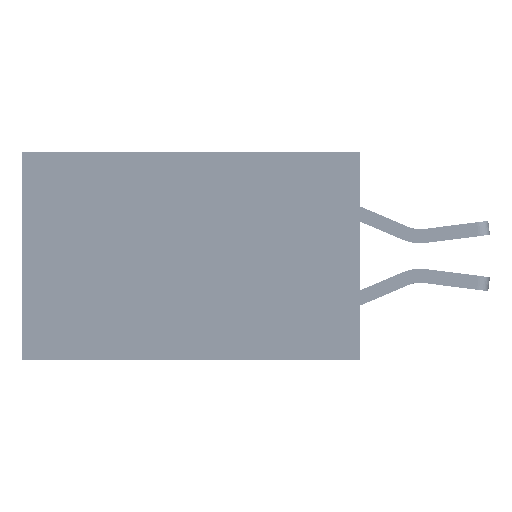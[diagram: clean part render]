
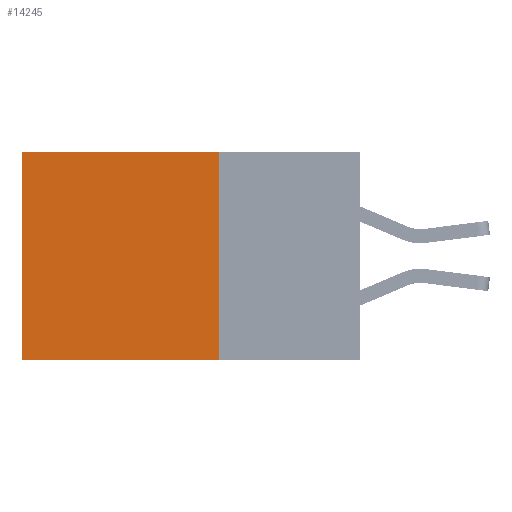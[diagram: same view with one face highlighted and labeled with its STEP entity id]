
A CAD part, left-side view. The second image highlights one B-rep face of the part: STEP entity #14245.
In plain terms, the highlighted planar face has unit normal (-1, 0, 0).
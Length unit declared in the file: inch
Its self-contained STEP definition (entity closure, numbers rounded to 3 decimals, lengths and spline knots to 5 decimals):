
#894 = VERTEX_POINT ( 'NONE', #29877 ) ;
#2317 = DIRECTION ( 'NONE',  ( 0., 1., 0. ) ) ;
#5609 = EDGE_CURVE ( 'NONE', #894, #10453, #28375, .T. ) ;
#5979 = CARTESIAN_POINT ( 'NONE',  ( 0.2875, 0.25, 0. ) ) ;
#8077 = DIRECTION ( 'NONE',  ( 0., 0., -1. ) ) ;
#8150 = DIRECTION ( 'NONE',  ( 0., 0., -1. ) ) ;
#8217 = PLANE ( 'NONE',  #35666 ) ;
#10453 = VERTEX_POINT ( 'NONE', #11294 ) ;
#11294 = CARTESIAN_POINT ( 'NONE',  ( 0.2875, 0.6, 0. ) ) ;
#11904 = EDGE_CURVE ( 'NONE', #894, #16902, #26312, .T. ) ;
#12482 = CARTESIAN_POINT ( 'NONE',  ( 0.2875, 0.25, -0.37 ) ) ;
#12704 = ORIENTED_EDGE ( 'NONE', *, *, #11904, .F. ) ;
#12740 = DIRECTION ( 'NONE',  ( 0., 1., 0. ) ) ;
#13519 = CARTESIAN_POINT ( 'NONE',  ( 0.2875, 0.25, 0. ) ) ;
#14245 = ADVANCED_FACE ( 'NONE', ( #19607 ), #8217, .F. ) ;
#15785 = VECTOR ( 'NONE', #35979, 39.37008 ) ;
#16902 = VERTEX_POINT ( 'NONE', #30801 ) ;
#19607 = FACE_OUTER_BOUND ( 'NONE', #24415, .T. ) ;
#19716 = ORIENTED_EDGE ( 'NONE', *, *, #25637, .T. ) ;
#20900 = ORIENTED_EDGE ( 'NONE', *, *, #34503, .F. ) ;
#23865 = VECTOR ( 'NONE', #12740, 39.37008 ) ;
#24415 = EDGE_LOOP ( 'NONE', ( #19716, #20900, #12704, #40371 ) ) ;
#24988 = CARTESIAN_POINT ( 'NONE',  ( 0.2875, 0.25, 0. ) ) ;
#25637 = EDGE_CURVE ( 'NONE', #10453, #33034, #28688, .T. ) ;
#26312 = LINE ( 'NONE', #13519, #15785 ) ;
#27309 = CARTESIAN_POINT ( 'NONE',  ( 0.2875, 0.6, 0. ) ) ;
#28375 = LINE ( 'NONE', #24988, #31819 ) ;
#28498 = DIRECTION ( 'NONE',  ( 1., 0., 0. ) ) ;
#28688 = LINE ( 'NONE', #27309, #35706 ) ;
#29877 = CARTESIAN_POINT ( 'NONE',  ( 0.2875, 0.25, 0. ) ) ;
#30801 = CARTESIAN_POINT ( 'NONE',  ( 0.2875, 0.25, -0.37 ) ) ;
#31819 = VECTOR ( 'NONE', #2317, 39.37008 ) ;
#32385 = LINE ( 'NONE', #12482, #23865 ) ;
#33034 = VERTEX_POINT ( 'NONE', #39414 ) ;
#34503 = EDGE_CURVE ( 'NONE', #16902, #33034, #32385, .T. ) ;
#35666 = AXIS2_PLACEMENT_3D ( 'NONE', #5979, #28498, #8077 ) ;
#35706 = VECTOR ( 'NONE', #8150, 39.37008 ) ;
#35979 = DIRECTION ( 'NONE',  ( 0., 0., -1. ) ) ;
#39414 = CARTESIAN_POINT ( 'NONE',  ( 0.2875, 0.6, -0.37 ) ) ;
#40371 = ORIENTED_EDGE ( 'NONE', *, *, #5609, .T. ) ;
